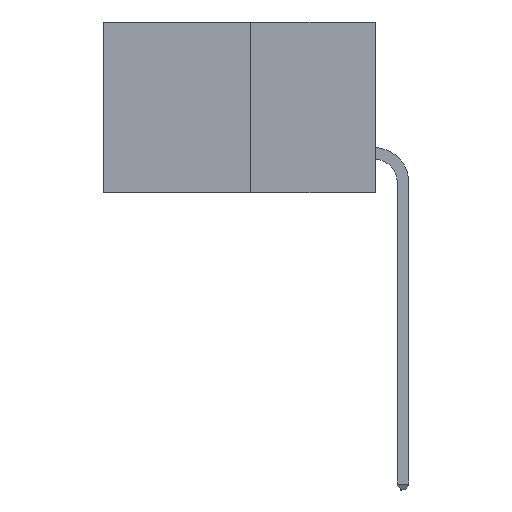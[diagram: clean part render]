
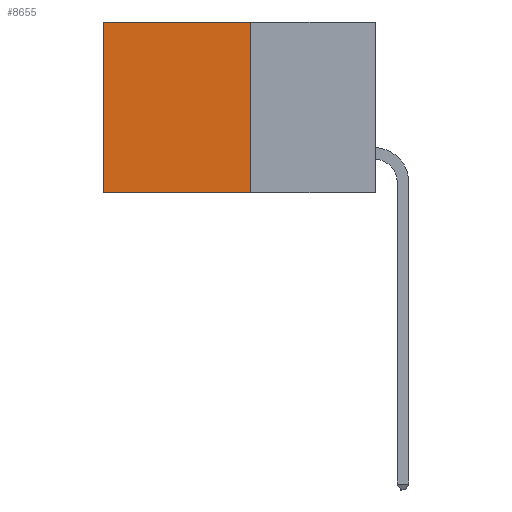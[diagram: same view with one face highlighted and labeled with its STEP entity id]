
A CAD part, left-side view. The second image highlights one B-rep face of the part: STEP entity #8655.
In plain terms, the highlighted planar face has unit normal (-1, 0, 0).
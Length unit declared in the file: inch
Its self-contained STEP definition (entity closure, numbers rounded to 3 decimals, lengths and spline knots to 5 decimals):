
#259 = CARTESIAN_POINT ( 'NONE',  ( 0.277, 0.59, -0.37 ) ) ;
#920 = PLANE ( 'NONE',  #3852 ) ;
#1117 = EDGE_LOOP ( 'NONE', ( #3219, #7133, #1353, #7860 ) ) ;
#1353 = ORIENTED_EDGE ( 'NONE', *, *, #2788, .F. ) ;
#2085 = DIRECTION ( 'NONE',  ( 0., 1., 0. ) ) ;
#2227 = VECTOR ( 'NONE', #11096, 39.37008 ) ;
#2304 = CARTESIAN_POINT ( 'NONE',  ( 0.277, 0.27, -0.37 ) ) ;
#2531 = CARTESIAN_POINT ( 'NONE',  ( 0.277, 0.27, 0. ) ) ;
#2788 = EDGE_CURVE ( 'NONE', #15053, #11463, #10640, .T. ) ;
#2976 = LINE ( 'NONE', #259, #10391 ) ;
#3219 = ORIENTED_EDGE ( 'NONE', *, *, #8935, .T. ) ;
#3236 = CARTESIAN_POINT ( 'NONE',  ( 0.277, 0.27, -0.37 ) ) ;
#3850 = EDGE_CURVE ( 'NONE', #15053, #11675, #10399, .T. ) ;
#3852 = AXIS2_PLACEMENT_3D ( 'NONE', #2304, #15216, #7675 ) ;
#4131 = VERTEX_POINT ( 'NONE', #10499 ) ;
#4180 = CARTESIAN_POINT ( 'NONE',  ( 0.277, 0.27, -0.37 ) ) ;
#5283 = FACE_OUTER_BOUND ( 'NONE', #1117, .T. ) ;
#6572 = CARTESIAN_POINT ( 'NONE',  ( 0.277, 0.27, -0.37 ) ) ;
#7133 = ORIENTED_EDGE ( 'NONE', *, *, #7276, .F. ) ;
#7276 = EDGE_CURVE ( 'NONE', #11463, #4131, #9687, .T. ) ;
#7675 = DIRECTION ( 'NONE',  ( 0., 0., -1. ) ) ;
#7860 = ORIENTED_EDGE ( 'NONE', *, *, #3850, .T. ) ;
#8655 = ADVANCED_FACE ( 'NONE', ( #5283 ), #920, .F. ) ;
#8707 = CARTESIAN_POINT ( 'NONE',  ( 0.277, 0.27, 0. ) ) ;
#8935 = EDGE_CURVE ( 'NONE', #11675, #4131, #2976, .T. ) ;
#9587 = DIRECTION ( 'NONE',  ( 0., 0., -1. ) ) ;
#9687 = LINE ( 'NONE', #3236, #2227 ) ;
#10006 = VECTOR ( 'NONE', #2085, 39.37008 ) ;
#10391 = VECTOR ( 'NONE', #9587, 39.37008 ) ;
#10399 = LINE ( 'NONE', #8707, #10006 ) ;
#10499 = CARTESIAN_POINT ( 'NONE',  ( 0.277, 0.59, -0.37 ) ) ;
#10640 = LINE ( 'NONE', #6572, #13586 ) ;
#11096 = DIRECTION ( 'NONE',  ( 0., 1., 0. ) ) ;
#11463 = VERTEX_POINT ( 'NONE', #4180 ) ;
#11675 = VERTEX_POINT ( 'NONE', #16130 ) ;
#13586 = VECTOR ( 'NONE', #15422, 39.37008 ) ;
#15053 = VERTEX_POINT ( 'NONE', #2531 ) ;
#15216 = DIRECTION ( 'NONE',  ( 1., 0., 0. ) ) ;
#15422 = DIRECTION ( 'NONE',  ( 0., 0., -1. ) ) ;
#16130 = CARTESIAN_POINT ( 'NONE',  ( 0.277, 0.59, 0. ) ) ;
